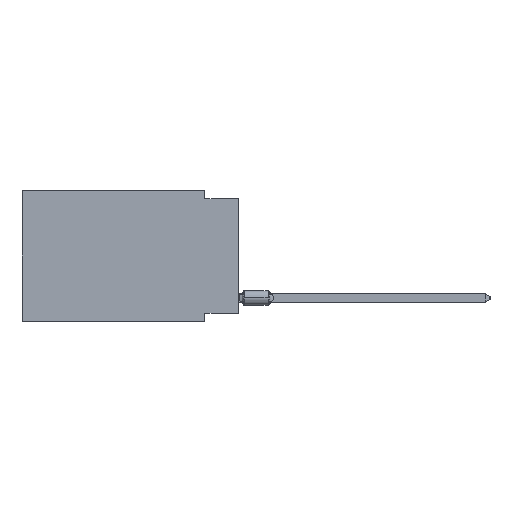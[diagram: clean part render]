
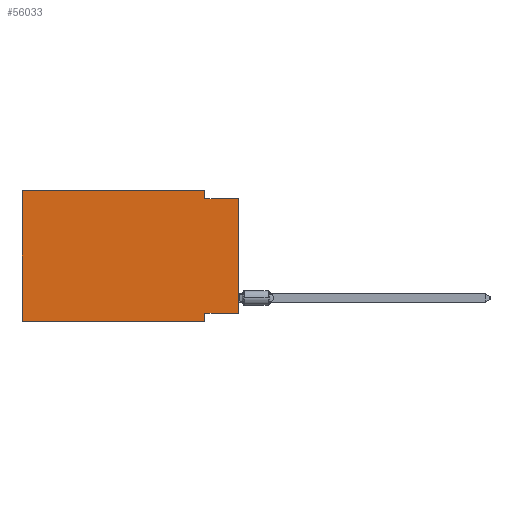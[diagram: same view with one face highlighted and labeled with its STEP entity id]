
A CAD part, left-side view. The second image highlights one B-rep face of the part: STEP entity #56033.
In plain terms, the highlighted planar face has unit normal (-1, 0, 0).
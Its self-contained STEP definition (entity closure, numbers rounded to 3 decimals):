
#655 = CARTESIAN_POINT ( 'NONE',  ( 0., 16.383, 0. ) ) ;
#809 = CARTESIAN_POINT ( 'NONE',  ( 0., 2.54, 0. ) ) ;
#872 = ORIENTED_EDGE ( 'NONE', *, *, #25121, .F. ) ;
#1231 = CARTESIAN_POINT ( 'NONE',  ( 0., 2.54, -9.906 ) ) ;
#1615 = VECTOR ( 'NONE', #30539, 1000. ) ;
#1698 = CARTESIAN_POINT ( 'NONE',  ( 0., 2.54, 0. ) ) ;
#2490 = DIRECTION ( 'NONE',  ( 0., -1., 0. ) ) ;
#5173 = DIRECTION ( 'NONE',  ( 0., 0., -1. ) ) ;
#5549 = CARTESIAN_POINT ( 'NONE',  ( 0., 16.383, -9.906 ) ) ;
#6017 = ORIENTED_EDGE ( 'NONE', *, *, #58260, .T. ) ;
#6397 = VECTOR ( 'NONE', #10970, 1000. ) ;
#7014 = LINE ( 'NONE', #29089, #58608 ) ;
#8301 = CARTESIAN_POINT ( 'NONE',  ( 0., 0., -0.635 ) ) ;
#9825 = CARTESIAN_POINT ( 'NONE',  ( 0., 16.383, 0. ) ) ;
#10441 = VERTEX_POINT ( 'NONE', #21600 ) ;
#10889 = ORIENTED_EDGE ( 'NONE', *, *, #16462, .F. ) ;
#10970 = DIRECTION ( 'NONE',  ( 0., -1., 0. ) ) ;
#11494 = CARTESIAN_POINT ( 'NONE',  ( 0., 0., -0.635 ) ) ;
#12273 = VECTOR ( 'NONE', #30475, 1000. ) ;
#15260 = LINE ( 'NONE', #9825, #12273 ) ;
#15528 = CARTESIAN_POINT ( 'NONE',  ( 0., 2.54, -0.635 ) ) ;
#16462 = EDGE_CURVE ( 'NONE', #28315, #10441, #41274, .T. ) ;
#21557 = EDGE_CURVE ( 'NONE', #54271, #33207, #27283, .T. ) ;
#21600 = CARTESIAN_POINT ( 'NONE',  ( 0., 2.54, -9.271 ) ) ;
#21825 = VERTEX_POINT ( 'NONE', #15528 ) ;
#22577 = VERTEX_POINT ( 'NONE', #1698 ) ;
#25121 = EDGE_CURVE ( 'NONE', #21825, #54803, #64083, .T. ) ;
#26673 = AXIS2_PLACEMENT_3D ( 'NONE', #655, #50649, #67338 ) ;
#27283 = LINE ( 'NONE', #5549, #6397 ) ;
#27943 = VECTOR ( 'NONE', #64102, 1000. ) ;
#28177 = PLANE ( 'NONE',  #26673 ) ;
#28315 = VERTEX_POINT ( 'NONE', #66506 ) ;
#29089 = CARTESIAN_POINT ( 'NONE',  ( 0., 2.54, -9.906 ) ) ;
#30152 = DIRECTION ( 'NONE',  ( 0., 0., -1. ) ) ;
#30475 = DIRECTION ( 'NONE',  ( 0., -1., 0. ) ) ;
#30539 = DIRECTION ( 'NONE',  ( 0., 0., 1. ) ) ;
#31038 = EDGE_CURVE ( 'NONE', #61143, #22577, #15260, .T. ) ;
#32914 = ORIENTED_EDGE ( 'NONE', *, *, #45394, .F. ) ;
#33207 = VERTEX_POINT ( 'NONE', #1231 ) ;
#33544 = ORIENTED_EDGE ( 'NONE', *, *, #49321, .F. ) ;
#35947 = CARTESIAN_POINT ( 'NONE',  ( 0., 0., 0. ) ) ;
#38051 = CARTESIAN_POINT ( 'NONE',  ( 0., 16.383, -9.906 ) ) ;
#39060 = CARTESIAN_POINT ( 'NONE',  ( 0., 16.383, 0. ) ) ;
#41274 = LINE ( 'NONE', #52871, #27943 ) ;
#41780 = ORIENTED_EDGE ( 'NONE', *, *, #45091, .F. ) ;
#45091 = EDGE_CURVE ( 'NONE', #54271, #61143, #63546, .T. ) ;
#45394 = EDGE_CURVE ( 'NONE', #22577, #21825, #50083, .T. ) ;
#46516 = CARTESIAN_POINT ( 'NONE',  ( 0., 16.383, 0. ) ) ;
#49321 = EDGE_CURVE ( 'NONE', #10441, #33207, #7014, .T. ) ;
#50083 = LINE ( 'NONE', #809, #69963 ) ;
#50545 = VECTOR ( 'NONE', #2490, 1000. ) ;
#50649 = DIRECTION ( 'NONE',  ( 1., 0., 0. ) ) ;
#52579 = ORIENTED_EDGE ( 'NONE', *, *, #31038, .F. ) ;
#52636 = DIRECTION ( 'NONE',  ( 0., 0., 1. ) ) ;
#52871 = CARTESIAN_POINT ( 'NONE',  ( 0., 0., -9.271 ) ) ;
#53709 = LINE ( 'NONE', #35947, #70733 ) ;
#54271 = VERTEX_POINT ( 'NONE', #38051 ) ;
#54803 = VERTEX_POINT ( 'NONE', #11494 ) ;
#55344 = EDGE_LOOP ( 'NONE', ( #6017, #872, #32914, #52579, #41780, #66031, #33544, #10889 ) ) ;
#56033 = ADVANCED_FACE ( 'NONE', ( #71005 ), #28177, .F. ) ;
#58260 = EDGE_CURVE ( 'NONE', #28315, #54803, #53709, .T. ) ;
#58608 = VECTOR ( 'NONE', #30152, 1000. ) ;
#61143 = VERTEX_POINT ( 'NONE', #39060 ) ;
#63546 = LINE ( 'NONE', #46516, #1615 ) ;
#64083 = LINE ( 'NONE', #8301, #50545 ) ;
#64102 = DIRECTION ( 'NONE',  ( 0., 1., 0. ) ) ;
#66031 = ORIENTED_EDGE ( 'NONE', *, *, #21557, .T. ) ;
#66506 = CARTESIAN_POINT ( 'NONE',  ( 0., 0., -9.271 ) ) ;
#67338 = DIRECTION ( 'NONE',  ( 0., 0., -1. ) ) ;
#69963 = VECTOR ( 'NONE', #5173, 1000. ) ;
#70733 = VECTOR ( 'NONE', #52636, 1000. ) ;
#71005 = FACE_OUTER_BOUND ( 'NONE', #55344, .T. ) ;
